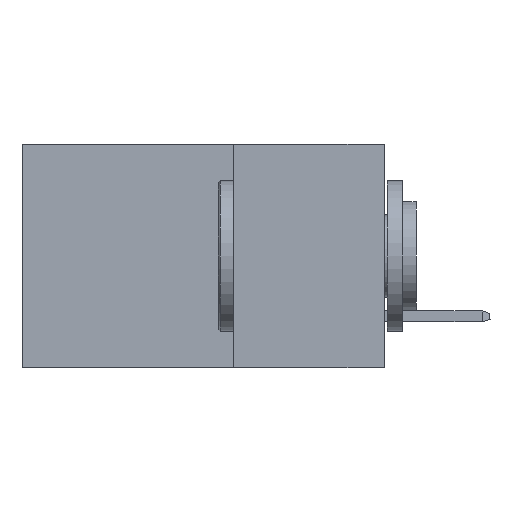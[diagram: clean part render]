
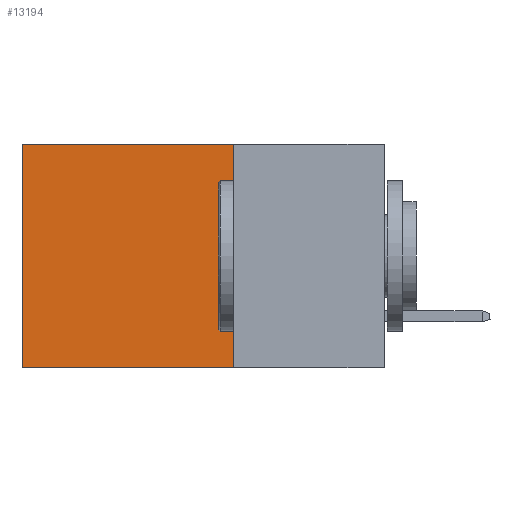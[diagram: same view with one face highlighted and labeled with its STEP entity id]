
A CAD part, left-side view. The second image highlights one B-rep face of the part: STEP entity #13194.
In plain terms, the highlighted planar face has unit normal (-1, 0, 0).
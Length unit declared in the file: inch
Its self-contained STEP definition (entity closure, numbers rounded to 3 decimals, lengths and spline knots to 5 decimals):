
#745 = DIRECTION ( 'NONE',  ( 0., 0., -1. ) ) ;
#1623 = CARTESIAN_POINT ( 'NONE',  ( 0.298, 0.25, -0.37 ) ) ;
#3920 = LINE ( 'NONE', #25058, #18924 ) ;
#5526 = VERTEX_POINT ( 'NONE', #18711 ) ;
#6142 = EDGE_CURVE ( 'NONE', #26571, #11024, #16842, .T. ) ;
#6673 = ORIENTED_EDGE ( 'NONE', *, *, #28683, .F. ) ;
#9220 = LINE ( 'NONE', #18513, #14088 ) ;
#9425 = CARTESIAN_POINT ( 'NONE',  ( 0.298, 0.6, -0.37 ) ) ;
#9614 = PLANE ( 'NONE',  #17759 ) ;
#11024 = VERTEX_POINT ( 'NONE', #9425 ) ;
#11313 = VERTEX_POINT ( 'NONE', #26358 ) ;
#11346 = CARTESIAN_POINT ( 'NONE',  ( 0.298, 0.25, -0.37 ) ) ;
#11582 = DIRECTION ( 'NONE',  ( 0., 1., 0. ) ) ;
#11834 = DIRECTION ( 'NONE',  ( 1., 0., 0. ) ) ;
#13194 = ADVANCED_FACE ( 'NONE', ( #20662 ), #9614, .F. ) ;
#13580 = DIRECTION ( 'NONE',  ( 0., 1., 0. ) ) ;
#13582 = LINE ( 'NONE', #16604, #20942 ) ;
#14088 = VECTOR ( 'NONE', #11582, 39.37008 ) ;
#16604 = CARTESIAN_POINT ( 'NONE',  ( 0.298, 0.6, 0. ) ) ;
#16842 = LINE ( 'NONE', #11346, #22083 ) ;
#17759 = AXIS2_PLACEMENT_3D ( 'NONE', #25185, #11834, #27425 ) ;
#17774 = ORIENTED_EDGE ( 'NONE', *, *, #6142, .F. ) ;
#18513 = CARTESIAN_POINT ( 'NONE',  ( 0.298, 0.25, 0. ) ) ;
#18711 = CARTESIAN_POINT ( 'NONE',  ( 0.298, 0.25, 0. ) ) ;
#18924 = VECTOR ( 'NONE', #745, 39.37008 ) ;
#20662 = FACE_OUTER_BOUND ( 'NONE', #25892, .T. ) ;
#20942 = VECTOR ( 'NONE', #23323, 39.37008 ) ;
#21306 = ORIENTED_EDGE ( 'NONE', *, *, #21395, .T. ) ;
#21395 = EDGE_CURVE ( 'NONE', #5526, #11313, #9220, .T. ) ;
#22083 = VECTOR ( 'NONE', #13580, 39.37008 ) ;
#23323 = DIRECTION ( 'NONE',  ( 0., 0., -1. ) ) ;
#24922 = EDGE_CURVE ( 'NONE', #11313, #11024, #13582, .T. ) ;
#24950 = ORIENTED_EDGE ( 'NONE', *, *, #24922, .T. ) ;
#25058 = CARTESIAN_POINT ( 'NONE',  ( 0.298, 0.25, 0. ) ) ;
#25185 = CARTESIAN_POINT ( 'NONE',  ( 0.298, 0.25, 0. ) ) ;
#25892 = EDGE_LOOP ( 'NONE', ( #24950, #17774, #6673, #21306 ) ) ;
#26358 = CARTESIAN_POINT ( 'NONE',  ( 0.298, 0.6, 0. ) ) ;
#26571 = VERTEX_POINT ( 'NONE', #1623 ) ;
#27425 = DIRECTION ( 'NONE',  ( 0., 0., -1. ) ) ;
#28683 = EDGE_CURVE ( 'NONE', #5526, #26571, #3920, .T. ) ;
